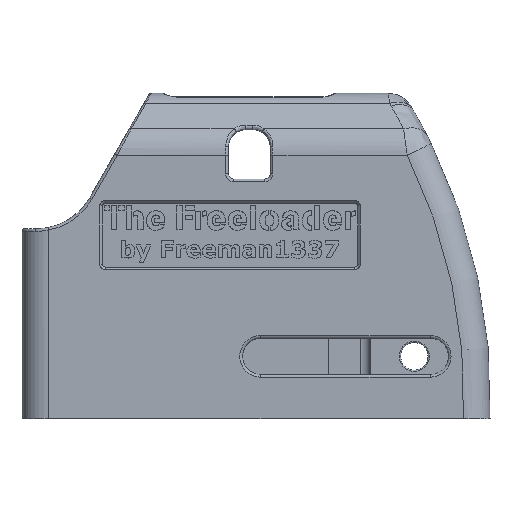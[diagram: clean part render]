
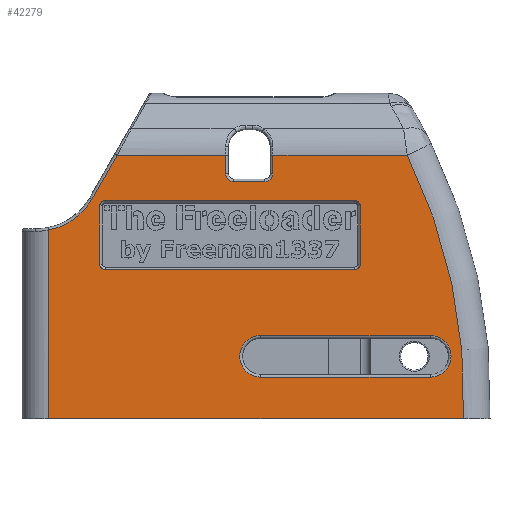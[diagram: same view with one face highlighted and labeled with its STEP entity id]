
A CAD part, left-side view. The second image highlights one B-rep face of the part: STEP entity #42279.
In plain terms, the highlighted planar face has unit normal (-1, 0, 0).
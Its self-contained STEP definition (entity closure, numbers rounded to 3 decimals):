
#4675=FACE_BOUND('',#15617,.T.);
#4676=FACE_BOUND('',#15618,.T.);
#5390=PLANE('',#44444);
#5566=LINE('',#51490,#8661);
#6174=LINE('',#54663,#9269);
#6179=LINE('',#54677,#9274);
#6183=LINE('',#54689,#9278);
#6187=LINE('',#54701,#9282);
#7534=LINE('',#74027,#10629);
#7537=LINE('',#74042,#10632);
#7541=LINE('',#74067,#10636);
#7542=LINE('',#74070,#10637);
#7543=LINE('',#74074,#10638);
#7544=LINE('',#74076,#10639);
#7545=LINE('',#74080,#10640);
#7546=LINE('',#74084,#10641);
#7547=LINE('',#74085,#10642);
#8661=VECTOR('',#45124,10.);
#9269=VECTOR('',#46176,10.);
#9274=VECTOR('',#46189,10.);
#9278=VECTOR('',#46201,10.);
#9282=VECTOR('',#46213,10.);
#10629=VECTOR('',#49122,10.);
#10632=VECTOR('',#49139,10.);
#10636=VECTOR('',#49157,10.);
#10637=VECTOR('',#49160,10.);
#10638=VECTOR('',#49163,10.);
#10639=VECTOR('',#49164,10.);
#10640=VECTOR('',#49167,10.);
#10641=VECTOR('',#49170,10.);
#10642=VECTOR('',#49171,10.);
#13152=FACE_OUTER_BOUND('',#15616,.T.);
#15616=EDGE_LOOP('',(#35698,#35699,#35700,#35701,#35702,#35703,#35704,#35705,
#35706,#35707,#35708,#35709));
#15617=EDGE_LOOP('',(#35710,#35711,#35712,#35713,#35714,#35715,#35716,#35717));
#15618=EDGE_LOOP('',(#35718,#35719,#35720,#35721));
#16812=CIRCLE('',#43639,1.);
#16814=CIRCLE('',#43643,1.);
#16816=CIRCLE('',#43647,1.);
#16818=CIRCLE('',#43651,1.);
#16978=CIRCLE('',#44435,3.925);
#16981=CIRCLE('',#44440,3.925);
#16983=CIRCLE('',#44445,12.);
#16984=CIRCLE('',#44446,103.5);
#16985=CIRCLE('',#44447,1.5);
#16986=CIRCLE('',#44448,1.5);
#17176=VERTEX_POINT('',#51469);
#17178=VERTEX_POINT('',#51489);
#17767=VERTEX_POINT('',#54660);
#17768=VERTEX_POINT('',#54662);
#17771=VERTEX_POINT('',#54669);
#17773=VERTEX_POINT('',#54675);
#17775=VERTEX_POINT('',#54681);
#17777=VERTEX_POINT('',#54687);
#17779=VERTEX_POINT('',#54693);
#17781=VERTEX_POINT('',#54699);
#20348=VERTEX_POINT('',#74024);
#20349=VERTEX_POINT('',#74026);
#20351=VERTEX_POINT('',#74032);
#20353=VERTEX_POINT('',#74038);
#20357=VERTEX_POINT('',#74065);
#20358=VERTEX_POINT('',#74066);
#20359=VERTEX_POINT('',#74068);
#20360=VERTEX_POINT('',#74071);
#20361=VERTEX_POINT('',#74073);
#20362=VERTEX_POINT('',#74075);
#20363=VERTEX_POINT('',#74077);
#20364=VERTEX_POINT('',#74079);
#20365=VERTEX_POINT('',#74081);
#20366=VERTEX_POINT('',#74083);
#21494=EDGE_CURVE('',#17178,#17176,#5566,.F.);
#22352=EDGE_CURVE('',#17768,#17767,#6174,.T.);
#22356=EDGE_CURVE('',#17767,#17771,#16812,.T.);
#22359=EDGE_CURVE('',#17771,#17773,#6179,.T.);
#22362=EDGE_CURVE('',#17773,#17775,#16814,.T.);
#22365=EDGE_CURVE('',#17775,#17777,#6183,.T.);
#22368=EDGE_CURVE('',#17777,#17779,#16816,.T.);
#22371=EDGE_CURVE('',#17779,#17781,#6187,.T.);
#22373=EDGE_CURVE('',#17781,#17768,#16818,.T.);
#25817=EDGE_CURVE('',#20348,#20349,#7534,.T.);
#25822=EDGE_CURVE('',#20349,#20351,#16978,.T.);
#25825=EDGE_CURVE('',#20351,#20353,#7537,.T.);
#25827=EDGE_CURVE('',#20353,#20348,#16981,.T.);
#25833=EDGE_CURVE('',#20357,#20358,#7541,.T.);
#25834=EDGE_CURVE('',#20359,#20357,#16983,.T.);
#25835=EDGE_CURVE('',#17178,#20359,#7542,.T.);
#25836=EDGE_CURVE('',#20360,#17176,#16984,.T.);
#25837=EDGE_CURVE('',#20360,#20361,#7543,.T.);
#25838=EDGE_CURVE('',#20362,#20361,#7544,.T.);
#25839=EDGE_CURVE('',#20363,#20362,#16985,.T.);
#25840=EDGE_CURVE('',#20364,#20363,#7545,.T.);
#25841=EDGE_CURVE('',#20365,#20364,#16986,.T.);
#25842=EDGE_CURVE('',#20366,#20365,#7546,.T.);
#25843=EDGE_CURVE('',#20366,#20358,#7547,.T.);
#35698=ORIENTED_EDGE('',*,*,#25833,.F.);
#35699=ORIENTED_EDGE('',*,*,#25834,.F.);
#35700=ORIENTED_EDGE('',*,*,#25835,.F.);
#35701=ORIENTED_EDGE('',*,*,#21494,.T.);
#35702=ORIENTED_EDGE('',*,*,#25836,.F.);
#35703=ORIENTED_EDGE('',*,*,#25837,.T.);
#35704=ORIENTED_EDGE('',*,*,#25838,.F.);
#35705=ORIENTED_EDGE('',*,*,#25839,.F.);
#35706=ORIENTED_EDGE('',*,*,#25840,.F.);
#35707=ORIENTED_EDGE('',*,*,#25841,.F.);
#35708=ORIENTED_EDGE('',*,*,#25842,.F.);
#35709=ORIENTED_EDGE('',*,*,#25843,.T.);
#35710=ORIENTED_EDGE('',*,*,#22352,.T.);
#35711=ORIENTED_EDGE('',*,*,#22356,.T.);
#35712=ORIENTED_EDGE('',*,*,#22359,.T.);
#35713=ORIENTED_EDGE('',*,*,#22362,.T.);
#35714=ORIENTED_EDGE('',*,*,#22365,.T.);
#35715=ORIENTED_EDGE('',*,*,#22368,.T.);
#35716=ORIENTED_EDGE('',*,*,#22371,.T.);
#35717=ORIENTED_EDGE('',*,*,#22373,.T.);
#35718=ORIENTED_EDGE('',*,*,#25817,.F.);
#35719=ORIENTED_EDGE('',*,*,#25827,.F.);
#35720=ORIENTED_EDGE('',*,*,#25825,.F.);
#35721=ORIENTED_EDGE('',*,*,#25822,.F.);
#42279=ADVANCED_FACE('',(#13152,#4675,#4676),#5390,.F.);
#43639=AXIS2_PLACEMENT_3D('',#54671,#46182,#46183);
#43643=AXIS2_PLACEMENT_3D('',#54683,#46194,#46195);
#43647=AXIS2_PLACEMENT_3D('',#54695,#46206,#46207);
#43651=AXIS2_PLACEMENT_3D('',#54704,#46217,#46218);
#44435=AXIS2_PLACEMENT_3D('',#74036,#49132,#49133);
#44440=AXIS2_PLACEMENT_3D('',#74045,#49144,#49145);
#44444=AXIS2_PLACEMENT_3D('',#74064,#49155,#49156);
#44445=AXIS2_PLACEMENT_3D('',#74069,#49158,#49159);
#44446=AXIS2_PLACEMENT_3D('',#74072,#49161,#49162);
#44447=AXIS2_PLACEMENT_3D('',#74078,#49165,#49166);
#44448=AXIS2_PLACEMENT_3D('',#74082,#49168,#49169);
#45124=DIRECTION('',(0.,1.,0.));
#46176=DIRECTION('',(0.,0.,1.));
#46182=DIRECTION('center_axis',(1.,0.,0.));
#46183=DIRECTION('ref_axis',(0.,0.,
1.));
#46189=DIRECTION('',(0.,-1.,0.));
#46194=DIRECTION('center_axis',(1.,0.,0.));
#46195=DIRECTION('ref_axis',(0.,-1.,0.));
#46201=DIRECTION('',(0.,0.,-1.));
#46206=DIRECTION('center_axis',(1.,0.,0.));
#46207=DIRECTION('ref_axis',(0.,0.,
-1.));
#46213=DIRECTION('',(0.,1.,0.));
#46217=DIRECTION('center_axis',(1.,0.,0.));
#46218=DIRECTION('ref_axis',(0.,1.,0.));
#49122=DIRECTION('',(0.,-1.,0.));
#49132=DIRECTION('center_axis',(-1.,0.,0.));
#49133=DIRECTION('ref_axis',(0.,-1.,0.));
#49139=DIRECTION('',(0.,1.,0.));
#49144=DIRECTION('center_axis',(-1.,0.,0.));
#49145=DIRECTION('ref_axis',(0.,1.,0.));
#49155=DIRECTION('center_axis',(1.,0.,0.));
#49156=DIRECTION('ref_axis',(0.,0.,-1.));
#49157=DIRECTION('',(0.,-0.499,0.866));
#49158=DIRECTION('center_axis',(-1.,0.,0.));
#49159=DIRECTION('ref_axis',(0.,-0.583,-0.812));
#49160=DIRECTION('',(0.,0.,1.));
#49161=DIRECTION('center_axis',(1.,0.,0.));
#49162=DIRECTION('ref_axis',(0.,-0.976,0.216));
#49163=DIRECTION('',(0.,1.,0.));
#49164=DIRECTION('',(0.,0.,1.));
#49165=DIRECTION('center_axis',(-1.,0.,0.));
#49166=DIRECTION('ref_axis',(0.,-0.707,-0.707));
#49167=DIRECTION('',(0.,-1.,0.));
#49168=DIRECTION('center_axis',(-1.,0.,0.));
#49169=DIRECTION('ref_axis',(0.,0.707,-0.707));
#49170=DIRECTION('',(0.,0.,-1.));
#49171=DIRECTION('',(0.,1.,0.));
#51469=CARTESIAN_POINT('',(-118.44,-51.472,-20.259));
#51489=CARTESIAN_POINT('',(-118.44,26.734,-20.259));
#51490=CARTESIAN_POINT('',(-118.44,-6.203,-20.259));
#54660=CARTESIAN_POINT('',(-118.44,17.053,19.853));
#54662=CARTESIAN_POINT('',(-118.44,17.053,8.817));
#54663=CARTESIAN_POINT('',(-118.44,17.053,8.815));
#54669=CARTESIAN_POINT('',(-118.44,16.053,20.853));
#54671=CARTESIAN_POINT('Origin',(-118.44,16.053,19.853));
#54675=CARTESIAN_POINT('',(-118.44,-31.007,20.853));
#54677=CARTESIAN_POINT('',(-118.44,1.824,20.853));
#54681=CARTESIAN_POINT('',(-118.44,-32.007,19.853));
#54683=CARTESIAN_POINT('Origin',(-118.44,-31.007,19.853));
#54687=CARTESIAN_POINT('',(-118.44,-32.007,8.817));
#54689=CARTESIAN_POINT('',(-118.44,-32.007,14.333));
#54693=CARTESIAN_POINT('',(-118.44,-31.007,7.817));
#54695=CARTESIAN_POINT('Origin',(-118.44,-31.007,8.817));
#54699=CARTESIAN_POINT('',(-118.44,16.053,7.817));
#54701=CARTESIAN_POINT('',(-118.44,-21.706,7.817));
#54704=CARTESIAN_POINT('Origin',(-118.44,16.053,8.817));
#74024=CARTESIAN_POINT('',(-118.44,-13.233,-12.45));
#74026=CARTESIAN_POINT('',(-118.44,-45.212,-12.45));
#74027=CARTESIAN_POINT('',(-118.44,-12.819,-12.45));
#74032=CARTESIAN_POINT('',(-118.44,-45.212,-4.6));
#74036=CARTESIAN_POINT('Origin',(-118.44,-45.212,-8.525));
#74038=CARTESIAN_POINT('',(-118.44,-13.233,-4.6));
#74042=CARTESIAN_POINT('',(-118.44,-12.819,-4.6));
#74045=CARTESIAN_POINT('Origin',(-118.44,-13.233,-8.525));
#74064=CARTESIAN_POINT('Origin',(-118.44,-12.406,8.812));
#74065=CARTESIAN_POINT('',(-118.44,18.591,21.057));
#74066=CARTESIAN_POINT('',(-118.44,13.797,29.372));
#74067=CARTESIAN_POINT('',(-118.44,11.452,33.44));
#74068=CARTESIAN_POINT('',(-118.44,26.734,15.264));
#74069=CARTESIAN_POINT('Origin',(-118.44,28.987,27.051));
#74070=CARTESIAN_POINT('',(-118.44,26.734,14.575));
#74071=CARTESIAN_POINT('',(-118.44,-40.894,29.372));
#74072=CARTESIAN_POINT('Origin',(-118.44,51.954,-16.36));
#74073=CARTESIAN_POINT('',(-118.44,-15.567,29.372));
#74074=CARTESIAN_POINT('',(-118.44,-56.546,29.372));
#74075=CARTESIAN_POINT('',(-118.44,-15.567,25.905));
#74076=CARTESIAN_POINT('',(-118.44,-15.567,16.859));
#74077=CARTESIAN_POINT('',(-118.44,-14.067,24.405));
#74078=CARTESIAN_POINT('Origin',(-118.44,-14.067,25.905));
#74079=CARTESIAN_POINT('',(-118.44,-8.167,24.405));
#74080=CARTESIAN_POINT('',(-118.44,-9.786,24.405));
#74081=CARTESIAN_POINT('',(-118.44,-6.667,25.905));
#74082=CARTESIAN_POINT('Origin',(-118.44,-8.167,25.905));
#74083=CARTESIAN_POINT('',(-118.44,-6.667,29.372));
#74084=CARTESIAN_POINT('',(-118.44,-6.667,19.859));
#74085=CARTESIAN_POINT('',(-118.44,-56.546,29.372));
